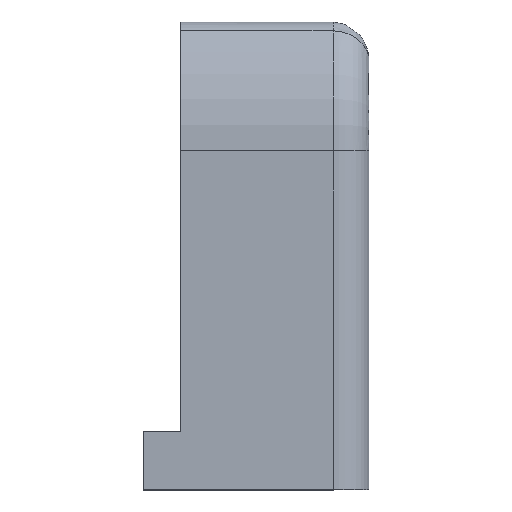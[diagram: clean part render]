
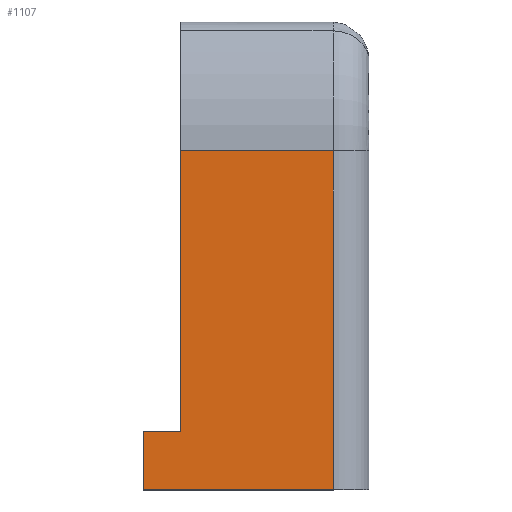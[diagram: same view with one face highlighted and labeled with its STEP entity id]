
A CAD part, top view. The second image highlights one B-rep face of the part: STEP entity #1107.
In plain terms, the highlighted planar face has unit normal (0, 0, 1).
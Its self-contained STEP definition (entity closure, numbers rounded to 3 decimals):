
#27 = DIRECTION ( 'NONE',  ( 0., 1., 0. ) ) ;
#50 = ORIENTED_EDGE ( 'NONE', *, *, #504, .F. ) ;
#103 = LINE ( 'NONE', #1312, #1117 ) ;
#128 = ORIENTED_EDGE ( 'NONE', *, *, #774, .T. ) ;
#176 = LINE ( 'NONE', #1699, #665 ) ;
#429 = CARTESIAN_POINT ( 'NONE',  ( 32.528, 40.065, 18.535 ) ) ;
#456 = VERTEX_POINT ( 'NONE', #1546 ) ;
#504 = EDGE_CURVE ( 'NONE', #1290, #925, #1205, .T. ) ;
#505 = ORIENTED_EDGE ( 'NONE', *, *, #1806, .T. ) ;
#536 = VECTOR ( 'NONE', #1329, 1000. ) ;
#577 = DIRECTION ( 'NONE',  ( 1., 0., 0. ) ) ;
#592 = ORIENTED_EDGE ( 'NONE', *, *, #670, .F. ) ;
#605 = CARTESIAN_POINT ( 'NONE',  ( 28.511, 36.937, 18.535 ) ) ;
#621 = CARTESIAN_POINT ( 'NONE',  ( 28.511, 0.06, 18.535 ) ) ;
#660 = DIRECTION ( 'NONE',  ( -1., 0., 0. ) ) ;
#665 = VECTOR ( 'NONE', #27, 1000. ) ;
#670 = EDGE_CURVE ( 'NONE', #1731, #1290, #103, .T. ) ;
#682 = VECTOR ( 'NONE', #577, 1000. ) ;
#693 = AXIS2_PLACEMENT_3D ( 'NONE', #429, #752, #1038 ) ;
#730 = LINE ( 'NONE', #1940, #682 ) ;
#752 = DIRECTION ( 'NONE',  ( 0., 0., 1. ) ) ;
#774 = EDGE_CURVE ( 'NONE', #1731, #1819, #946, .T. ) ;
#925 = VERTEX_POINT ( 'NONE', #1371 ) ;
#926 = CARTESIAN_POINT ( 'NONE',  ( 11.9, 36.937, 18.535 ) ) ;
#946 = LINE ( 'NONE', #1629, #536 ) ;
#1026 = CARTESIAN_POINT ( 'NONE',  ( 7.8, 6.41, 18.535 ) ) ;
#1038 = DIRECTION ( 'NONE',  ( 0., -1., 0. ) ) ;
#1107 = ADVANCED_FACE ( 'NONE', ( #1423 ), #1934, .T. ) ;
#1112 = LINE ( 'NONE', #1816, #1835 ) ;
#1117 = VECTOR ( 'NONE', #1763, 1000. ) ;
#1119 = EDGE_LOOP ( 'NONE', ( #1848, #505, #50, #592, #128, #1229 ) ) ;
#1176 = VECTOR ( 'NONE', #660, 1000. ) ;
#1205 = LINE ( 'NONE', #1854, #1176 ) ;
#1206 = VERTEX_POINT ( 'NONE', #1026 ) ;
#1229 = ORIENTED_EDGE ( 'NONE', *, *, #1882, .F. ) ;
#1290 = VERTEX_POINT ( 'NONE', #621 ) ;
#1312 = CARTESIAN_POINT ( 'NONE',  ( 28.511, 39.937, 18.535 ) ) ;
#1329 = DIRECTION ( 'NONE',  ( -1., 0., 0. ) ) ;
#1371 = CARTESIAN_POINT ( 'NONE',  ( 7.8, 0.06, 18.535 ) ) ;
#1423 = FACE_OUTER_BOUND ( 'NONE', #1119, .T. ) ;
#1453 = EDGE_CURVE ( 'NONE', #1206, #456, #730, .T. ) ;
#1546 = CARTESIAN_POINT ( 'NONE',  ( 11.9, 6.41, 18.535 ) ) ;
#1629 = CARTESIAN_POINT ( 'NONE',  ( 22.114, 36.937, 18.535 ) ) ;
#1699 = CARTESIAN_POINT ( 'NONE',  ( 11.9, 28.237, 18.535 ) ) ;
#1731 = VERTEX_POINT ( 'NONE', #605 ) ;
#1763 = DIRECTION ( 'NONE',  ( 0., -1., 0. ) ) ;
#1806 = EDGE_CURVE ( 'NONE', #1206, #925, #1112, .T. ) ;
#1816 = CARTESIAN_POINT ( 'NONE',  ( 7.8, 23.729, 18.535 ) ) ;
#1819 = VERTEX_POINT ( 'NONE', #926 ) ;
#1835 = VECTOR ( 'NONE', #1944, 1000. ) ;
#1848 = ORIENTED_EDGE ( 'NONE', *, *, #1453, .F. ) ;
#1854 = CARTESIAN_POINT ( 'NONE',  ( 32.528, 0.06, 18.535 ) ) ;
#1882 = EDGE_CURVE ( 'NONE', #456, #1819, #176, .T. ) ;
#1934 = PLANE ( 'NONE',  #693 ) ;
#1940 = CARTESIAN_POINT ( 'NONE',  ( 5.35, 6.41, 18.535 ) ) ;
#1944 = DIRECTION ( 'NONE',  ( 0., -1., 0. ) ) ;
